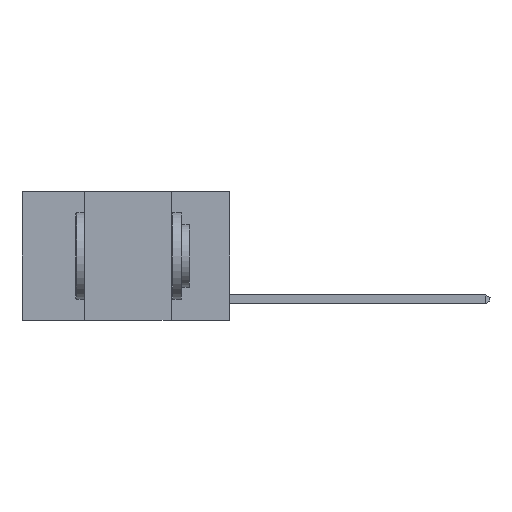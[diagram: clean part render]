
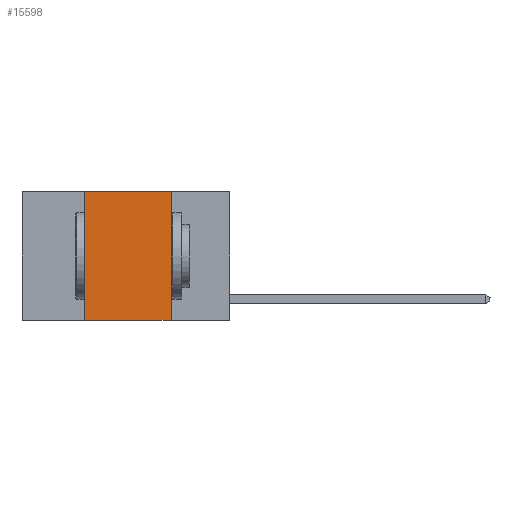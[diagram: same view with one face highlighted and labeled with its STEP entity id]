
A CAD part, left-side view. The second image highlights one B-rep face of the part: STEP entity #15598.
In plain terms, the highlighted planar face has unit normal (-1, 0, 0).
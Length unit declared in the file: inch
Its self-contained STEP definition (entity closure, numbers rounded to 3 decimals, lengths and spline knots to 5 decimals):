
#1036 = CARTESIAN_POINT ( 'NONE',  ( 0., 0.6, 0. ) ) ;
#2158 = DIRECTION ( 'NONE',  ( 0., -1., 0. ) ) ;
#2770 = CARTESIAN_POINT ( 'NONE',  ( 0., 0.42, 0. ) ) ;
#2867 = LINE ( 'NONE', #3246, #4522 ) ;
#3246 = CARTESIAN_POINT ( 'NONE',  ( 0., 0.17, 0. ) ) ;
#4522 = VECTOR ( 'NONE', #18236, 39.37008 ) ;
#4890 = DIRECTION ( 'NONE',  ( 0., -1., 0. ) ) ;
#4917 = ORIENTED_EDGE ( 'NONE', *, *, #17186, .F. ) ;
#5444 = VECTOR ( 'NONE', #4890, 39.37008 ) ;
#5584 = VERTEX_POINT ( 'NONE', #15589 ) ;
#6351 = CARTESIAN_POINT ( 'NONE',  ( 0., 0.17, 0. ) ) ;
#6934 = CARTESIAN_POINT ( 'NONE',  ( 0., 0.6, 0. ) ) ;
#7411 = PLANE ( 'NONE',  #22644 ) ;
#8366 = VERTEX_POINT ( 'NONE', #6351 ) ;
#8915 = DIRECTION ( 'NONE',  ( 0., 0., 1. ) ) ;
#9286 = ORIENTED_EDGE ( 'NONE', *, *, #24545, .F. ) ;
#10194 = VERTEX_POINT ( 'NONE', #24448 ) ;
#10802 = VECTOR ( 'NONE', #8915, 39.37008 ) ;
#10883 = EDGE_CURVE ( 'NONE', #10194, #5584, #21109, .T. ) ;
#12143 = EDGE_LOOP ( 'NONE', ( #9286, #4917, #15036, #13043 ) ) ;
#13043 = ORIENTED_EDGE ( 'NONE', *, *, #10883, .T. ) ;
#15036 = ORIENTED_EDGE ( 'NONE', *, *, #22666, .F. ) ;
#15125 = CARTESIAN_POINT ( 'NONE',  ( 0., 0.42, 0. ) ) ;
#15589 = CARTESIAN_POINT ( 'NONE',  ( 0., 0.17, -0.37 ) ) ;
#15598 = ADVANCED_FACE ( 'NONE', ( #20614 ), #7411, .F. ) ;
#16532 = VECTOR ( 'NONE', #2158, 39.37008 ) ;
#17186 = EDGE_CURVE ( 'NONE', #18937, #8366, #22151, .T. ) ;
#18236 = DIRECTION ( 'NONE',  ( 0., 0., -1. ) ) ;
#18457 = DIRECTION ( 'NONE',  ( 1., 0., 0. ) ) ;
#18706 = DIRECTION ( 'NONE',  ( 0., 0., -1. ) ) ;
#18937 = VERTEX_POINT ( 'NONE', #15125 ) ;
#20010 = LINE ( 'NONE', #2770, #10802 ) ;
#20614 = FACE_OUTER_BOUND ( 'NONE', #12143, .T. ) ;
#21109 = LINE ( 'NONE', #23073, #16532 ) ;
#22151 = LINE ( 'NONE', #6934, #5444 ) ;
#22644 = AXIS2_PLACEMENT_3D ( 'NONE', #1036, #18457, #18706 ) ;
#22666 = EDGE_CURVE ( 'NONE', #10194, #18937, #20010, .T. ) ;
#23073 = CARTESIAN_POINT ( 'NONE',  ( 0., 0.6, -0.37 ) ) ;
#24448 = CARTESIAN_POINT ( 'NONE',  ( 0., 0.42, -0.37 ) ) ;
#24545 = EDGE_CURVE ( 'NONE', #8366, #5584, #2867, .T. ) ;
